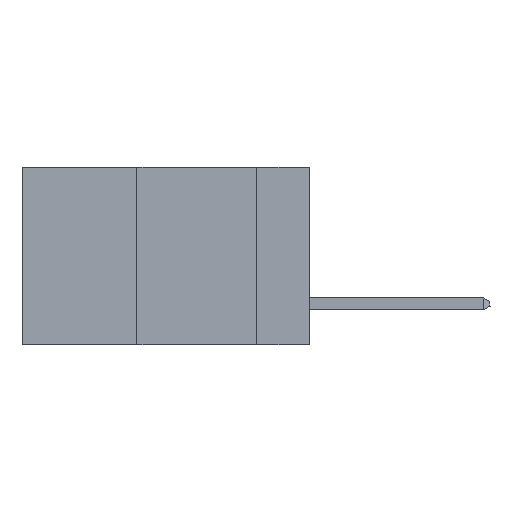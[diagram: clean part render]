
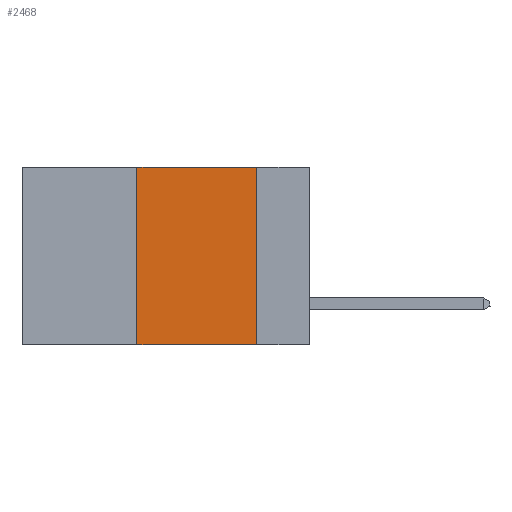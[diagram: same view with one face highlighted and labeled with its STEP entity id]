
A CAD part, left-side view. The second image highlights one B-rep face of the part: STEP entity #2468.
In plain terms, the highlighted planar face has unit normal (-1, 0, 0).
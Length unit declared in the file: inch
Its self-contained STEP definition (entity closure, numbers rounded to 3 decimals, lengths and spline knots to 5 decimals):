
#20 = VECTOR ( 'NONE', #38, 39.37008 ) ;
#38 = DIRECTION ( 'NONE',  ( 0., 0., -1. ) ) ;
#1111 = LINE ( 'NONE', #10955, #4414 ) ;
#1284 = CARTESIAN_POINT ( 'NONE',  ( 0., 0.36, 0. ) ) ;
#1315 = DIRECTION ( 'NONE',  ( 0., 0., -1. ) ) ;
#1363 = CARTESIAN_POINT ( 'NONE',  ( 0., 0.6, 0. ) ) ;
#2124 = CARTESIAN_POINT ( 'NONE',  ( 0., 0.11, 0. ) ) ;
#2348 = EDGE_CURVE ( 'NONE', #10159, #5540, #8957, .T. ) ;
#2468 = ADVANCED_FACE ( 'NONE', ( #3784 ), #9401, .F. ) ;
#2543 = VERTEX_POINT ( 'NONE', #12586 ) ;
#2695 = EDGE_CURVE ( 'NONE', #2543, #5866, #7026, .T. ) ;
#3256 = DIRECTION ( 'NONE',  ( 1., 0., 0. ) ) ;
#3572 = CARTESIAN_POINT ( 'NONE',  ( 0., 0.11, -0.37 ) ) ;
#3753 = DIRECTION ( 'NONE',  ( 0., 0., 1. ) ) ;
#3784 = FACE_OUTER_BOUND ( 'NONE', #8210, .T. ) ;
#4073 = VECTOR ( 'NONE', #8614, 39.37008 ) ;
#4414 = VECTOR ( 'NONE', #4661, 39.37008 ) ;
#4661 = DIRECTION ( 'NONE',  ( 0., -1., 0. ) ) ;
#4805 = CARTESIAN_POINT ( 'NONE',  ( 0., 0.11, 0. ) ) ;
#5540 = VERTEX_POINT ( 'NONE', #3572 ) ;
#5866 = VERTEX_POINT ( 'NONE', #1284 ) ;
#7026 = LINE ( 'NONE', #10841, #11380 ) ;
#7557 = ORIENTED_EDGE ( 'NONE', *, *, #8534, .F. ) ;
#7622 = ORIENTED_EDGE ( 'NONE', *, *, #9794, .T. ) ;
#8210 = EDGE_LOOP ( 'NONE', ( #8760, #7557, #12161, #7622 ) ) ;
#8534 = EDGE_CURVE ( 'NONE', #5866, #10159, #1111, .T. ) ;
#8614 = DIRECTION ( 'NONE',  ( 0., -1., 0. ) ) ;
#8760 = ORIENTED_EDGE ( 'NONE', *, *, #2348, .F. ) ;
#8957 = LINE ( 'NONE', #2124, #20 ) ;
#9401 = PLANE ( 'NONE',  #12675 ) ;
#9689 = CARTESIAN_POINT ( 'NONE',  ( 0., 0.6, -0.37 ) ) ;
#9794 = EDGE_CURVE ( 'NONE', #2543, #5540, #11498, .T. ) ;
#10159 = VERTEX_POINT ( 'NONE', #4805 ) ;
#10841 = CARTESIAN_POINT ( 'NONE',  ( 0., 0.36, 0. ) ) ;
#10955 = CARTESIAN_POINT ( 'NONE',  ( 0., 0.6, 0. ) ) ;
#11380 = VECTOR ( 'NONE', #3753, 39.37008 ) ;
#11498 = LINE ( 'NONE', #9689, #4073 ) ;
#12161 = ORIENTED_EDGE ( 'NONE', *, *, #2695, .F. ) ;
#12586 = CARTESIAN_POINT ( 'NONE',  ( 0., 0.36, -0.37 ) ) ;
#12675 = AXIS2_PLACEMENT_3D ( 'NONE', #1363, #3256, #1315 ) ;
